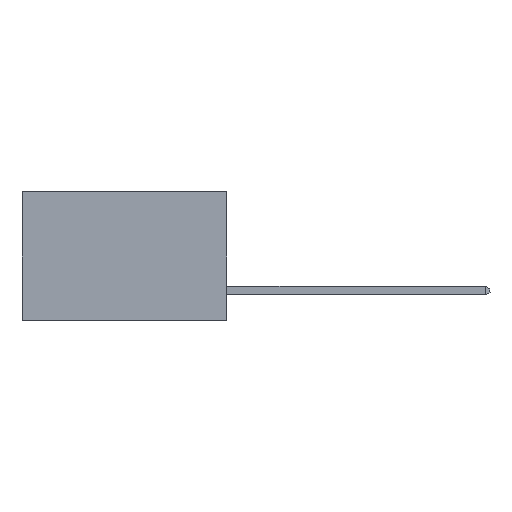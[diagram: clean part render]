
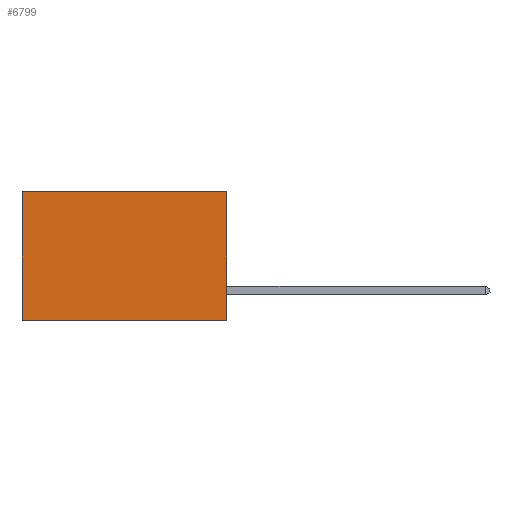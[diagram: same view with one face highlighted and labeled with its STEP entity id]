
A CAD part, left-side view. The second image highlights one B-rep face of the part: STEP entity #6799.
In plain terms, the highlighted planar face has unit normal (-1, 0, 0).
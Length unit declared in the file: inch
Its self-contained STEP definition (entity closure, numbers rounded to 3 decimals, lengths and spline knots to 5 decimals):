
#650 = CARTESIAN_POINT ( 'NONE',  ( 0.277, 0., -0.37 ) ) ;
#930 = LINE ( 'NONE', #4250, #8222 ) ;
#1766 = VERTEX_POINT ( 'NONE', #6500 ) ;
#1854 = EDGE_CURVE ( 'NONE', #5217, #7199, #5683, .T. ) ;
#2240 = DIRECTION ( 'NONE',  ( 0., 1., 0. ) ) ;
#2370 = PLANE ( 'NONE',  #5317 ) ;
#2488 = EDGE_CURVE ( 'NONE', #1766, #7199, #930, .T. ) ;
#2598 = ORIENTED_EDGE ( 'NONE', *, *, #2488, .T. ) ;
#2883 = ORIENTED_EDGE ( 'NONE', *, *, #11702, .F. ) ;
#3204 = LINE ( 'NONE', #4962, #7892 ) ;
#3282 = VECTOR ( 'NONE', #2240, 39.37008 ) ;
#4240 = CARTESIAN_POINT ( 'NONE',  ( 0.277, 0., -0.37 ) ) ;
#4250 = CARTESIAN_POINT ( 'NONE',  ( 0.277, 0.59, -0.37 ) ) ;
#4629 = EDGE_LOOP ( 'NONE', ( #2598, #7571, #2883, #7865 ) ) ;
#4962 = CARTESIAN_POINT ( 'NONE',  ( 0.277, 0., -0.37 ) ) ;
#5193 = DIRECTION ( 'NONE',  ( 0., 0., -1. ) ) ;
#5217 = VERTEX_POINT ( 'NONE', #9253 ) ;
#5220 = DIRECTION ( 'NONE',  ( 0., 0., -1. ) ) ;
#5317 = AXIS2_PLACEMENT_3D ( 'NONE', #4240, #10601, #5193 ) ;
#5683 = LINE ( 'NONE', #650, #7867 ) ;
#5754 = CARTESIAN_POINT ( 'NONE',  ( 0.277, 0.59, -0.37 ) ) ;
#5808 = LINE ( 'NONE', #8752, #3282 ) ;
#5956 = DIRECTION ( 'NONE',  ( 0., 0., -1. ) ) ;
#6500 = CARTESIAN_POINT ( 'NONE',  ( 0.277, 0.59, 0. ) ) ;
#6799 = ADVANCED_FACE ( 'NONE', ( #11960 ), #2370, .F. ) ;
#7199 = VERTEX_POINT ( 'NONE', #5754 ) ;
#7571 = ORIENTED_EDGE ( 'NONE', *, *, #1854, .F. ) ;
#7865 = ORIENTED_EDGE ( 'NONE', *, *, #8269, .T. ) ;
#7867 = VECTOR ( 'NONE', #11893, 39.37008 ) ;
#7892 = VECTOR ( 'NONE', #5956, 39.37008 ) ;
#8222 = VECTOR ( 'NONE', #5220, 39.37008 ) ;
#8269 = EDGE_CURVE ( 'NONE', #11344, #1766, #5808, .T. ) ;
#8274 = CARTESIAN_POINT ( 'NONE',  ( 0.277, 0., 0. ) ) ;
#8752 = CARTESIAN_POINT ( 'NONE',  ( 0.277, 0., 0. ) ) ;
#9253 = CARTESIAN_POINT ( 'NONE',  ( 0.277, 0., -0.37 ) ) ;
#10601 = DIRECTION ( 'NONE',  ( 1., 0., 0. ) ) ;
#11344 = VERTEX_POINT ( 'NONE', #8274 ) ;
#11702 = EDGE_CURVE ( 'NONE', #11344, #5217, #3204, .T. ) ;
#11893 = DIRECTION ( 'NONE',  ( 0., 1., 0. ) ) ;
#11960 = FACE_OUTER_BOUND ( 'NONE', #4629, .T. ) ;
